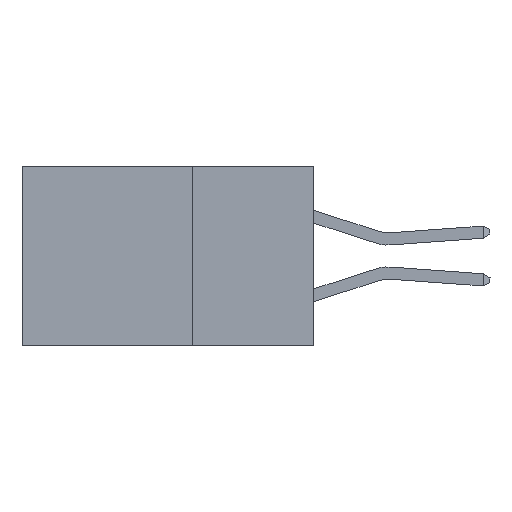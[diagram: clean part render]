
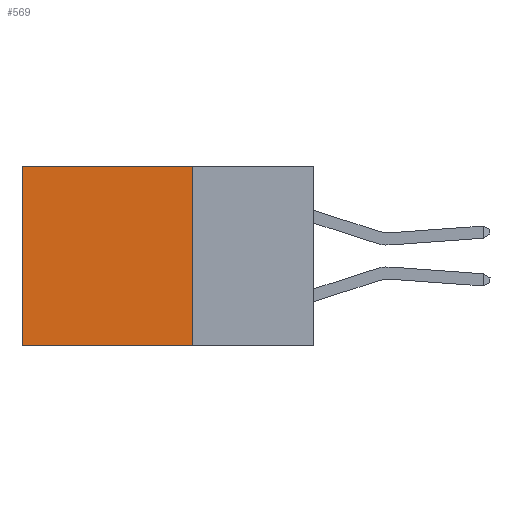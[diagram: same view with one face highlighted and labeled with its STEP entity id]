
A CAD part, left-side view. The second image highlights one B-rep face of the part: STEP entity #569.
In plain terms, the highlighted planar face has unit normal (-1, 0, 0).
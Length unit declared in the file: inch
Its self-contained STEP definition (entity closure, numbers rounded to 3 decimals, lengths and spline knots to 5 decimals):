
#569 = ADVANCED_FACE ( 'NONE', ( #4905 ), #17376, .F. ) ;
#999 = VECTOR ( 'NONE', #4734, 39.37008 ) ;
#1487 = VECTOR ( 'NONE', #11051, 39.37008 ) ;
#2038 = ORIENTED_EDGE ( 'NONE', *, *, #12892, .F. ) ;
#2089 = VERTEX_POINT ( 'NONE', #17581 ) ;
#2100 = ORIENTED_EDGE ( 'NONE', *, *, #17764, .T. ) ;
#2326 = VERTEX_POINT ( 'NONE', #4785 ) ;
#3469 = LINE ( 'NONE', #15460, #12099 ) ;
#3766 = EDGE_CURVE ( 'NONE', #12532, #2326, #11021, .T. ) ;
#4734 = DIRECTION ( 'NONE',  ( 0., 0., -1. ) ) ;
#4785 = CARTESIAN_POINT ( 'NONE',  ( 0.2875, 0.25, -0.37 ) ) ;
#4905 = FACE_OUTER_BOUND ( 'NONE', #20100, .T. ) ;
#5287 = CARTESIAN_POINT ( 'NONE',  ( 0.2875, 0.25, 0. ) ) ;
#7050 = DIRECTION ( 'NONE',  ( 1., 0., 0. ) ) ;
#7416 = AXIS2_PLACEMENT_3D ( 'NONE', #8699, #7050, #19121 ) ;
#7740 = LINE ( 'NONE', #9317, #1487 ) ;
#8699 = CARTESIAN_POINT ( 'NONE',  ( 0.2875, 0.25, 0. ) ) ;
#9317 = CARTESIAN_POINT ( 'NONE',  ( 0.2875, 0.25, -0.37 ) ) ;
#9970 = CARTESIAN_POINT ( 'NONE',  ( 0.2875, 0.6, 0. ) ) ;
#10081 = CARTESIAN_POINT ( 'NONE',  ( 0.2875, 0.25, 0. ) ) ;
#11021 = LINE ( 'NONE', #5287, #11532 ) ;
#11051 = DIRECTION ( 'NONE',  ( 0., 1., 0. ) ) ;
#11532 = VECTOR ( 'NONE', #17348, 39.37008 ) ;
#12099 = VECTOR ( 'NONE', #13721, 39.37008 ) ;
#12532 = VERTEX_POINT ( 'NONE', #10081 ) ;
#12892 = EDGE_CURVE ( 'NONE', #2326, #2089, #7740, .T. ) ;
#13721 = DIRECTION ( 'NONE',  ( 0., 1., 0. ) ) ;
#14153 = ORIENTED_EDGE ( 'NONE', *, *, #3766, .F. ) ;
#14824 = LINE ( 'NONE', #9970, #999 ) ;
#15460 = CARTESIAN_POINT ( 'NONE',  ( 0.2875, 0.25, 0. ) ) ;
#15792 = ORIENTED_EDGE ( 'NONE', *, *, #19815, .T. ) ;
#17348 = DIRECTION ( 'NONE',  ( 0., 0., -1. ) ) ;
#17376 = PLANE ( 'NONE',  #7416 ) ;
#17581 = CARTESIAN_POINT ( 'NONE',  ( 0.2875, 0.6, -0.37 ) ) ;
#17764 = EDGE_CURVE ( 'NONE', #12532, #21336, #3469, .T. ) ;
#19121 = DIRECTION ( 'NONE',  ( 0., 0., -1. ) ) ;
#19122 = CARTESIAN_POINT ( 'NONE',  ( 0.2875, 0.6, 0. ) ) ;
#19815 = EDGE_CURVE ( 'NONE', #21336, #2089, #14824, .T. ) ;
#20100 = EDGE_LOOP ( 'NONE', ( #15792, #2038, #14153, #2100 ) ) ;
#21336 = VERTEX_POINT ( 'NONE', #19122 ) ;
